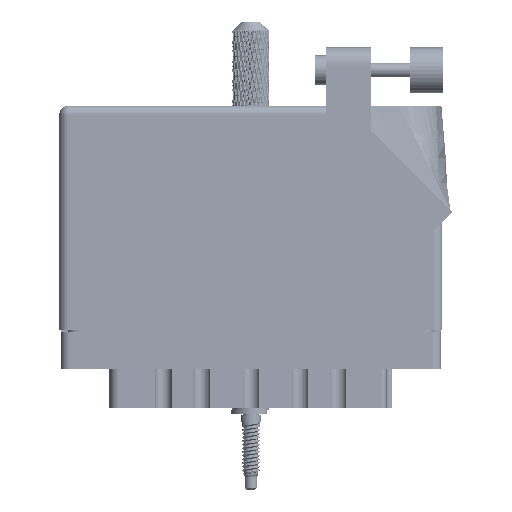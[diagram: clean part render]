
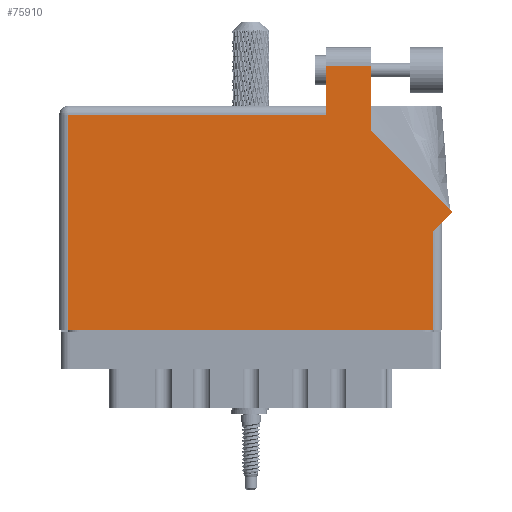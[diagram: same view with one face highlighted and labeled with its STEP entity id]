
A CAD part, front view. The second image highlights one B-rep face of the part: STEP entity #75910.
In plain terms, the highlighted face is planar.
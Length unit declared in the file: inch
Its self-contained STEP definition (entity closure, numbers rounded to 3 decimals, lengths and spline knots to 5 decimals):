
#66 = VERTEX_POINT ( 'NONE', #106691 ) ;
#461 = CARTESIAN_POINT ( 'NONE',  ( 2.126, 1.36442, 0. ) ) ;
#468 = CARTESIAN_POINT ( 'NONE',  ( 2.126, 1.805, 0. ) ) ;
#2182 = ORIENTED_EDGE ( 'NONE', *, *, #56670, .T. ) ;
#3913 = ORIENTED_EDGE ( 'NONE', *, *, #7560, .T. ) ;
#5542 = VERTEX_POINT ( 'NONE', #58867 ) ;
#7560 = EDGE_CURVE ( 'NONE', #60626, #7861, #49385, .T. ) ;
#7861 = VERTEX_POINT ( 'NONE', #63875 ) ;
#9999 = VECTOR ( 'NONE', #36737, 39.37008 ) ;
#10412 = VERTEX_POINT ( 'NONE', #90449 ) ;
#11848 = EDGE_CURVE ( 'NONE', #7861, #43906, #63067, .T. ) ;
#13872 = FACE_OUTER_BOUND ( 'NONE', #30047, .T. ) ;
#19102 = LINE ( 'NONE', #80528, #57954 ) ;
#19828 = DIRECTION ( 'NONE',  ( 0., -1., 0. ) ) ;
#20132 = LINE ( 'NONE', #461, #9999 ) ;
#22671 = DIRECTION ( 'NONE',  ( 0., 1., 0. ) ) ;
#27091 = ORIENTED_EDGE ( 'NONE', *, *, #87119, .T. ) ;
#30047 = EDGE_LOOP ( 'NONE', ( #115112, #3913, #70624, #60051, #112017, #81870, #51263, #2182, #27091 ) ) ;
#30084 = VECTOR ( 'NONE', #22671, 39.37008 ) ;
#31059 = CARTESIAN_POINT ( 'NONE',  ( 0.062, 0., 0. ) ) ;
#32543 = CARTESIAN_POINT ( 'NONE',  ( 1.819, 1.805, 0. ) ) ;
#36737 = DIRECTION ( 'NONE',  ( 0., 1., 0. ) ) ;
#40049 = LINE ( 'NONE', #61451, #78935 ) ;
#41881 = LINE ( 'NONE', #63510, #72002 ) ;
#42144 = LINE ( 'NONE', #31059, #76656 ) ;
#43906 = VERTEX_POINT ( 'NONE', #109763 ) ;
#45400 = DIRECTION ( 'NONE',  ( -1., 0., 0. ) ) ;
#49385 = LINE ( 'NONE', #32543, #104103 ) ;
#51263 = ORIENTED_EDGE ( 'NONE', *, *, #68488, .T. ) ;
#56507 = PLANE ( 'NONE',  #87120 ) ;
#56670 = EDGE_CURVE ( 'NONE', #66, #109050, #19102, .T. ) ;
#57954 = VECTOR ( 'NONE', #108311, 39.37008 ) ;
#58589 = LINE ( 'NONE', #111939, #80200 ) ;
#58867 = CARTESIAN_POINT ( 'NONE',  ( 2.55, 0., 0. ) ) ;
#60051 = ORIENTED_EDGE ( 'NONE', *, *, #85208, .T. ) ;
#60142 = VECTOR ( 'NONE', #19828, 39.37008 ) ;
#60626 = VERTEX_POINT ( 'NONE', #468 ) ;
#61451 = CARTESIAN_POINT ( 'NONE',  ( 2.68271, 0.80771, 0. ) ) ;
#63067 = LINE ( 'NONE', #93063, #60142 ) ;
#63510 = CARTESIAN_POINT ( 'NONE',  ( 0., 1.468, 0. ) ) ;
#63875 = CARTESIAN_POINT ( 'NONE',  ( 1.819, 1.805, 0. ) ) ;
#67951 = CARTESIAN_POINT ( 'NONE',  ( 0.062, 1.468, 0. ) ) ;
#68488 = EDGE_CURVE ( 'NONE', #5542, #66, #99176, .T. ) ;
#69565 = DIRECTION ( 'NONE',  ( -1., 0., 0. ) ) ;
#70624 = ORIENTED_EDGE ( 'NONE', *, *, #11848, .T. ) ;
#72002 = VECTOR ( 'NONE', #45400, 39.37008 ) ;
#75191 = EDGE_CURVE ( 'NONE', #112503, #5542, #58589, .T. ) ;
#75910 = ADVANCED_FACE ( 'NONE', ( #13872 ), #56507, .F. ) ;
#76656 = VECTOR ( 'NONE', #113173, 39.37008 ) ;
#78935 = VECTOR ( 'NONE', #108171, 39.37008 ) ;
#80200 = VECTOR ( 'NONE', #93850, 39.37008 ) ;
#80528 = CARTESIAN_POINT ( 'NONE',  ( 2.612, 0.737, 0. ) ) ;
#80551 = EDGE_CURVE ( 'NONE', #82241, #112503, #42144, .T. ) ;
#81870 = ORIENTED_EDGE ( 'NONE', *, *, #75191, .T. ) ;
#82241 = VERTEX_POINT ( 'NONE', #67951 ) ;
#83075 = CARTESIAN_POINT ( 'NONE',  ( 0., 1.53, 0. ) ) ;
#83856 = DIRECTION ( 'NONE',  ( 0., 0., -1. ) ) ;
#85208 = EDGE_CURVE ( 'NONE', #43906, #82241, #41881, .T. ) ;
#87043 = CARTESIAN_POINT ( 'NONE',  ( 2.55, 0.737, 0. ) ) ;
#87119 = EDGE_CURVE ( 'NONE', #109050, #10412, #40049, .T. ) ;
#87120 = AXIS2_PLACEMENT_3D ( 'NONE', #83075, #83856, #93545 ) ;
#90449 = CARTESIAN_POINT ( 'NONE',  ( 2.126, 1.36442, 0. ) ) ;
#93063 = CARTESIAN_POINT ( 'NONE',  ( 1.819, 1.53, 0. ) ) ;
#93545 = DIRECTION ( 'NONE',  ( -1., 0., 0. ) ) ;
#93850 = DIRECTION ( 'NONE',  ( 1., 0., 0. ) ) ;
#95914 = CARTESIAN_POINT ( 'NONE',  ( 2.68271, 0.80771, 0. ) ) ;
#98603 = CARTESIAN_POINT ( 'NONE',  ( 0.062, 0., 0. ) ) ;
#99176 = LINE ( 'NONE', #87043, #30084 ) ;
#104103 = VECTOR ( 'NONE', #69565, 39.37008 ) ;
#106691 = CARTESIAN_POINT ( 'NONE',  ( 2.55, 0.675, 0. ) ) ;
#108171 = DIRECTION ( 'NONE',  ( -0.707, 0.707, 0. ) ) ;
#108311 = DIRECTION ( 'NONE',  ( 0.707, 0.707, 0. ) ) ;
#109050 = VERTEX_POINT ( 'NONE', #95914 ) ;
#109763 = CARTESIAN_POINT ( 'NONE',  ( 1.819, 1.468, 0. ) ) ;
#111939 = CARTESIAN_POINT ( 'NONE',  ( 0., 0., 0. ) ) ;
#112017 = ORIENTED_EDGE ( 'NONE', *, *, #80551, .T. ) ;
#112503 = VERTEX_POINT ( 'NONE', #98603 ) ;
#113173 = DIRECTION ( 'NONE',  ( 0., -1., 0. ) ) ;
#115112 = ORIENTED_EDGE ( 'NONE', *, *, #115881, .T. ) ;
#115881 = EDGE_CURVE ( 'NONE', #10412, #60626, #20132, .T. ) ;
